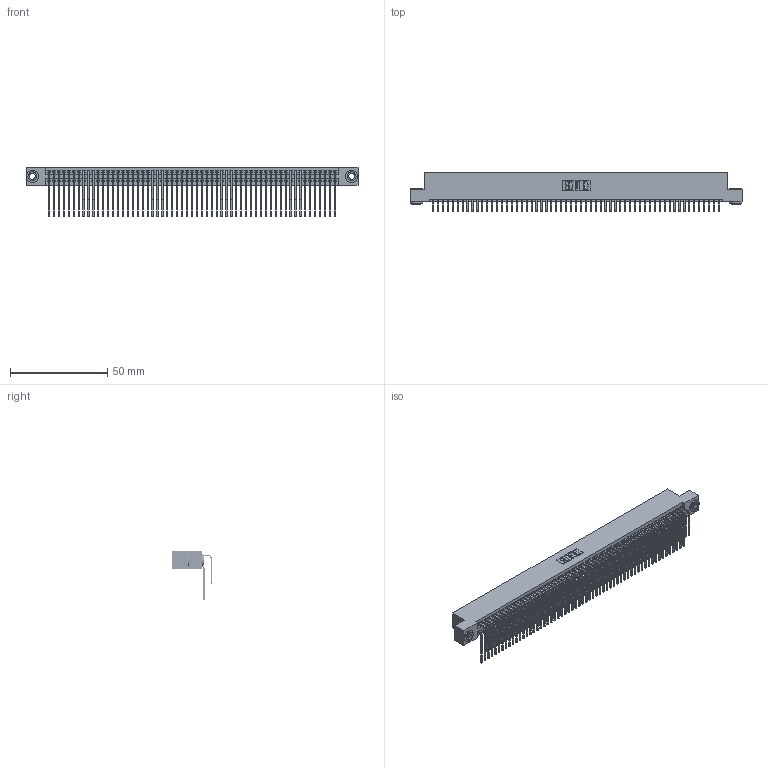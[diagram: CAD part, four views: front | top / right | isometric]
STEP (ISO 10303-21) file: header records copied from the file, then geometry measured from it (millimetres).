
FILE_DESCRIPTION (( 'STEP AP203' ), '1' );
FILE_NAME ('395-118-559-203.STEP', '2018-12-03T11:35:56', ( '' ), ( '' ), 'SwSTEP 2.0', 'SolidWorks 2016', '' );
FILE_SCHEMA (( 'CONFIG_CONTROL_DESIGN' ));
Length unit declared in the file: inch
Products named in the file (5): 395-118-559-203; 345-250-002_345-250-002-102; 345-292-001_559 Tail - 2; 345-292-001_558 559 Tail - 1; 345 Part_Flush Mounting Lugs - 0.156 Dia-TH
Assembly tree (121 placements, depth 2):
  395-118-559-203
    345 Part_Flush Mounting Lugs - 0.156 Dia-TH
    345-292-001_558 559 Tail - 1  x59
    345-292-001_559 Tail - 2  x59
    345-250-002_345-250-002-102  x2
Bounding box: 171.07 x 20.56 x 25.53 mm (x, y, z)
Volume: 17475.7 mm3; surface area: 29567.1 mm2
Topology: 121 solids, 121 shells, 6300 faces, 18707 edges, 12310 vertices
Faces by surface type: plane 4220, cylinder 2072, cone 8
Entity records: 46306 total; most frequent: CARTESIAN_POINT 7766, ORIENTED_EDGE 7642, DIRECTION 6831, EDGE_CURVE 3821, LINE 3389, VECTOR 3389, VERTEX_POINT 2542, AXIS2_PLACEMENT_3D 1721
